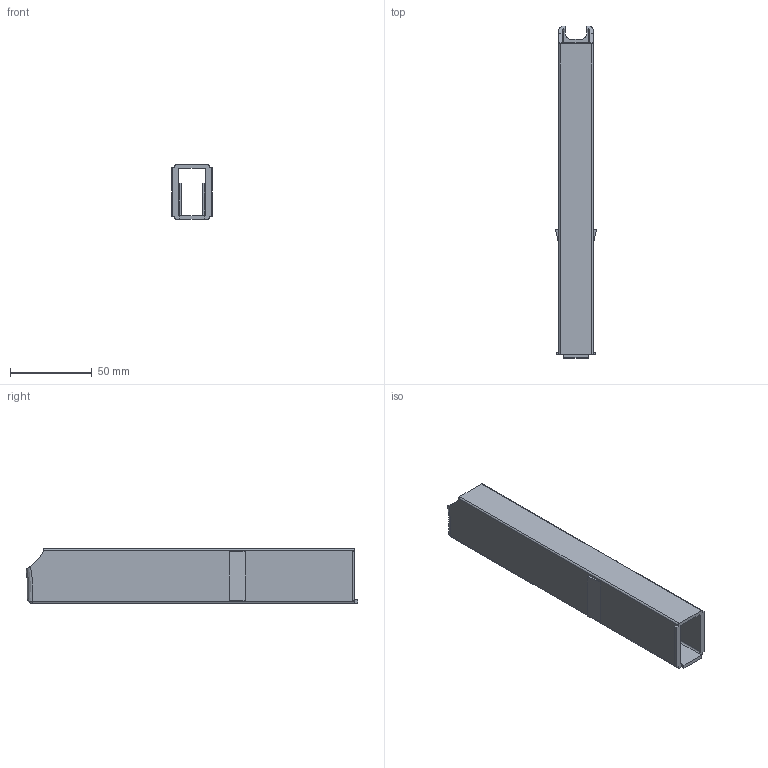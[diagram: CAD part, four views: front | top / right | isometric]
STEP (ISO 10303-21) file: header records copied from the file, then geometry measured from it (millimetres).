
FILE_DESCRIPTION (( 'STEP AP214' ), '1' );
FILE_NAME ('mag_body.STEP', '2013-06-02T20:15:27', ( '' ), ( '' ), 'SwSTEP 2.0', 'SolidWorks 2013', '' );
FILE_SCHEMA (( 'AUTOMOTIVE_DESIGN' ));
Length unit declared in the file: millimetre
Products named in the file (1): mag_body
Bounding box: 25 x 202.81 x 33.5 mm (x, y, z)
Volume: 41855.1 mm3; surface area: 39793.7 mm2
Topology: 1 solids, 1 shells, 213 faces, 582 edges, 380 vertices
Faces by surface type: plane 104, bspline 79, cylinder 26, sphere 2, torus 2
Entity records: 11710 total; most frequent: CARTESIAN_POINT 6825, ORIENTED_EDGE 1152, DIRECTION 728, EDGE_CURVE 576, VERTEX_POINT 378, VECTOR 362, LINE 362, EDGE_LOOP 240
